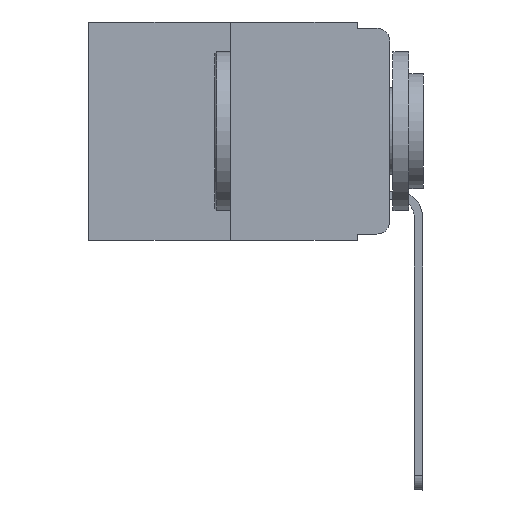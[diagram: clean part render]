
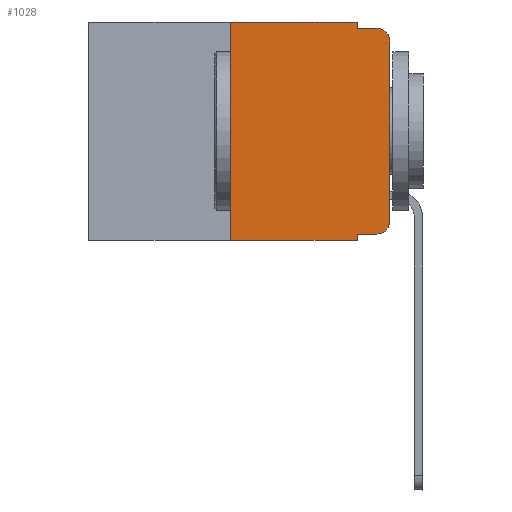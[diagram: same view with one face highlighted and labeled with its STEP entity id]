
A CAD part, left-side view. The second image highlights one B-rep face of the part: STEP entity #1028.
In plain terms, the highlighted planar face has unit normal (-1, 0, 0).
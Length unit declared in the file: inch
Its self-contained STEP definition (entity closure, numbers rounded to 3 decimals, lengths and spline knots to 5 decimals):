
#305 = VECTOR ( 'NONE', #12079, 39.37008 ) ;
#495 = DIRECTION ( 'NONE',  ( -1., 0., 0. ) ) ;
#593 = DIRECTION ( 'NONE',  ( 0., 0., -1. ) ) ;
#715 = LINE ( 'NONE', #19521, #19140 ) ;
#1028 = ADVANCED_FACE ( 'NONE', ( #13620 ), #2315, .F. ) ;
#1166 = LINE ( 'NONE', #18426, #305 ) ;
#1343 = ORIENTED_EDGE ( 'NONE', *, *, #9677, .T. ) ;
#1428 = ORIENTED_EDGE ( 'NONE', *, *, #18275, .T. ) ;
#1478 = CARTESIAN_POINT ( 'NONE',  ( 0., 0.051, 0. ) ) ;
#1720 = CARTESIAN_POINT ( 'NONE',  ( 0., 0., -0.03 ) ) ;
#1814 = ORIENTED_EDGE ( 'NONE', *, *, #15894, .F. ) ;
#2315 = PLANE ( 'NONE',  #15838 ) ;
#2486 = DIRECTION ( 'NONE',  ( 0., -1., 0. ) ) ;
#2828 = DIRECTION ( 'NONE',  ( 0., 0., 1. ) ) ;
#3832 = ORIENTED_EDGE ( 'NONE', *, *, #7398, .F. ) ;
#4342 = CARTESIAN_POINT ( 'NONE',  ( 0., 0.473, -0.343 ) ) ;
#4358 = CARTESIAN_POINT ( 'NONE',  ( 0., 0.051, 0. ) ) ;
#4391 = CARTESIAN_POINT ( 'NONE',  ( 0., 0.051, -0.333 ) ) ;
#5235 = DIRECTION ( 'NONE',  ( -1., 0., 0. ) ) ;
#5487 = CARTESIAN_POINT ( 'NONE',  ( 0., 0.473, 0. ) ) ;
#5602 = CARTESIAN_POINT ( 'NONE',  ( 0., 0.25, 0. ) ) ;
#5989 = LINE ( 'NONE', #4358, #8237 ) ;
#6207 = VECTOR ( 'NONE', #2486, 39.37008 ) ;
#6305 = VERTEX_POINT ( 'NONE', #14439 ) ;
#6440 = VERTEX_POINT ( 'NONE', #18100 ) ;
#6482 = ORIENTED_EDGE ( 'NONE', *, *, #7472, .F. ) ;
#6989 = DIRECTION ( 'NONE',  ( 0., 0., 1. ) ) ;
#7223 = VERTEX_POINT ( 'NONE', #19203 ) ;
#7302 = LINE ( 'NONE', #19623, #6207 ) ;
#7398 = EDGE_CURVE ( 'NONE', #17552, #15940, #8923, .T. ) ;
#7472 = EDGE_CURVE ( 'NONE', #6440, #6305, #16839, .T. ) ;
#7536 = VERTEX_POINT ( 'NONE', #4391 ) ;
#7779 = EDGE_CURVE ( 'NONE', #19209, #14550, #12169, .T. ) ;
#8237 = VECTOR ( 'NONE', #12085, 39.37008 ) ;
#8387 = CARTESIAN_POINT ( 'NONE',  ( 0., 0.051, -0.343 ) ) ;
#8414 = ORIENTED_EDGE ( 'NONE', *, *, #20322, .T. ) ;
#8895 = DIRECTION ( 'NONE',  ( 0., 0., -1. ) ) ;
#8923 = LINE ( 'NONE', #13249, #11549 ) ;
#9280 = ORIENTED_EDGE ( 'NONE', *, *, #9456, .T. ) ;
#9456 = EDGE_CURVE ( 'NONE', #7536, #7223, #7302, .T. ) ;
#9677 = EDGE_CURVE ( 'NONE', #10065, #6305, #20305, .T. ) ;
#10052 = DIRECTION ( 'NONE',  ( 0., -1., 0. ) ) ;
#10065 = VERTEX_POINT ( 'NONE', #1720 ) ;
#10615 = DIRECTION ( 'NONE',  ( 0., -1., 0. ) ) ;
#11104 = CARTESIAN_POINT ( 'NONE',  ( 0., 0.02, -0.03 ) ) ;
#11212 = DIRECTION ( 'NONE',  ( 0., 0., -1. ) ) ;
#11549 = VECTOR ( 'NONE', #10052, 39.37008 ) ;
#12079 = DIRECTION ( 'NONE',  ( 0., 0., -1. ) ) ;
#12085 = DIRECTION ( 'NONE',  ( 0., 0., -1. ) ) ;
#12169 = LINE ( 'NONE', #4342, #20104 ) ;
#12507 = ORIENTED_EDGE ( 'NONE', *, *, #7779, .T. ) ;
#12932 = EDGE_CURVE ( 'NONE', #19209, #17552, #15379, .T. ) ;
#13249 = CARTESIAN_POINT ( 'NONE',  ( 0., 0.473, 0. ) ) ;
#13467 = ORIENTED_EDGE ( 'NONE', *, *, #14682, .F. ) ;
#13620 = FACE_OUTER_BOUND ( 'NONE', #15027, .T. ) ;
#13959 = CARTESIAN_POINT ( 'NONE',  ( 0., 0.051, -0.01 ) ) ;
#14439 = CARTESIAN_POINT ( 'NONE',  ( 0., 0.02, -0.01 ) ) ;
#14550 = VERTEX_POINT ( 'NONE', #8387 ) ;
#14682 = EDGE_CURVE ( 'NONE', #15940, #6440, #1166, .T. ) ;
#15027 = EDGE_LOOP ( 'NONE', ( #8414, #1343, #6482, #13467, #3832, #20035, #12507, #1814, #9280, #1428 ) ) ;
#15196 = CIRCLE ( 'NONE', #18128, 0.02 ) ;
#15379 = LINE ( 'NONE', #5602, #18995 ) ;
#15838 = AXIS2_PLACEMENT_3D ( 'NONE', #5487, #18122, #8895 ) ;
#15894 = EDGE_CURVE ( 'NONE', #7536, #14550, #5989, .T. ) ;
#15940 = VERTEX_POINT ( 'NONE', #1478 ) ;
#16788 = CARTESIAN_POINT ( 'NONE',  ( 0., 0.25, 0. ) ) ;
#16839 = LINE ( 'NONE', #13959, #19410 ) ;
#17552 = VERTEX_POINT ( 'NONE', #16788 ) ;
#18100 = CARTESIAN_POINT ( 'NONE',  ( 0., 0.051, -0.01 ) ) ;
#18122 = DIRECTION ( 'NONE',  ( 1., 0., 0. ) ) ;
#18128 = AXIS2_PLACEMENT_3D ( 'NONE', #19204, #495, #593 ) ;
#18275 = EDGE_CURVE ( 'NONE', #7223, #18921, #15196, .T. ) ;
#18344 = CARTESIAN_POINT ( 'NONE',  ( 0., 0., -0.313 ) ) ;
#18426 = CARTESIAN_POINT ( 'NONE',  ( 0., 0.051, 0. ) ) ;
#18921 = VERTEX_POINT ( 'NONE', #18344 ) ;
#18995 = VECTOR ( 'NONE', #2828, 39.37008 ) ;
#19009 = AXIS2_PLACEMENT_3D ( 'NONE', #11104, #5235, #11212 ) ;
#19140 = VECTOR ( 'NONE', #6989, 39.37008 ) ;
#19203 = CARTESIAN_POINT ( 'NONE',  ( 0., 0.02, -0.333 ) ) ;
#19204 = CARTESIAN_POINT ( 'NONE',  ( 0., 0.02, -0.313 ) ) ;
#19209 = VERTEX_POINT ( 'NONE', #19327 ) ;
#19327 = CARTESIAN_POINT ( 'NONE',  ( 0., 0.25, -0.343 ) ) ;
#19410 = VECTOR ( 'NONE', #20203, 39.37008 ) ;
#19521 = CARTESIAN_POINT ( 'NONE',  ( 0., 0., 0. ) ) ;
#19623 = CARTESIAN_POINT ( 'NONE',  ( 0., 0.051, -0.333 ) ) ;
#20035 = ORIENTED_EDGE ( 'NONE', *, *, #12932, .F. ) ;
#20104 = VECTOR ( 'NONE', #10615, 39.37008 ) ;
#20203 = DIRECTION ( 'NONE',  ( 0., -1., 0. ) ) ;
#20305 = CIRCLE ( 'NONE', #19009, 0.02 ) ;
#20322 = EDGE_CURVE ( 'NONE', #18921, #10065, #715, .T. ) ;
